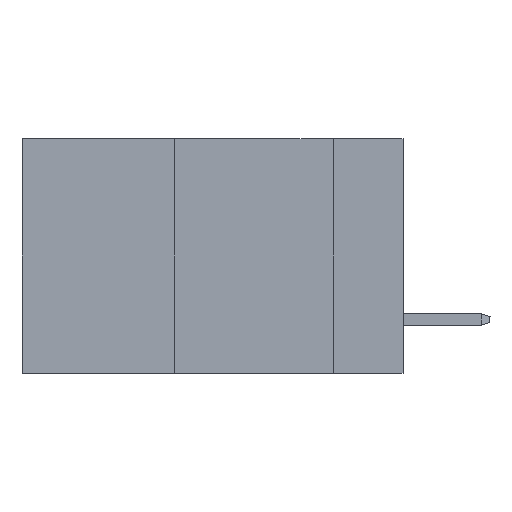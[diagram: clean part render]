
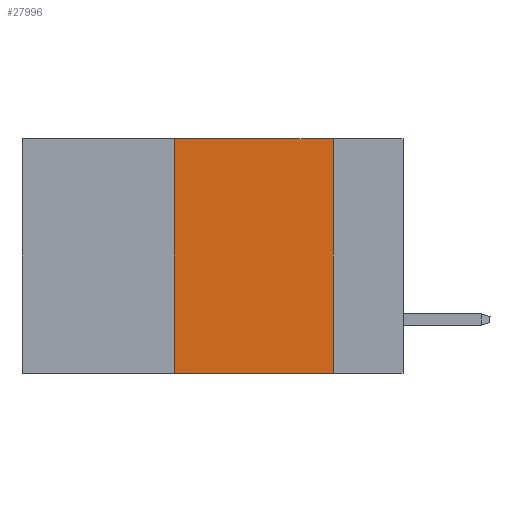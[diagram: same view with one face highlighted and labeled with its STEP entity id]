
A CAD part, left-side view. The second image highlights one B-rep face of the part: STEP entity #27996.
In plain terms, the highlighted planar face has unit normal (-1, 0, 0).
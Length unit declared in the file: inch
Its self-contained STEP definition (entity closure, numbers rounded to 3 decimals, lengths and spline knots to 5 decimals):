
#1361 = EDGE_CURVE ( 'NONE', #14462, #41740, #31360, .T. ) ;
#6105 = VECTOR ( 'NONE', #28665, 39.37008 ) ;
#7190 = LINE ( 'NONE', #13065, #34862 ) ;
#11686 = VECTOR ( 'NONE', #42303, 39.37008 ) ;
#12021 = EDGE_CURVE ( 'NONE', #26013, #41740, #7190, .T. ) ;
#13065 = CARTESIAN_POINT ( 'NONE',  ( 0., 0.6, -0.37 ) ) ;
#13126 = CARTESIAN_POINT ( 'NONE',  ( 0., 0.36, 0. ) ) ;
#14462 = VERTEX_POINT ( 'NONE', #42915 ) ;
#15807 = CARTESIAN_POINT ( 'NONE',  ( 0., 0.6, 0. ) ) ;
#17053 = CARTESIAN_POINT ( 'NONE',  ( 0., 0.36, 0. ) ) ;
#17493 = CARTESIAN_POINT ( 'NONE',  ( 0., 0.36, -0.37 ) ) ;
#18672 = CARTESIAN_POINT ( 'NONE',  ( 0., 0.11, -0.37 ) ) ;
#21296 = EDGE_CURVE ( 'NONE', #35274, #14462, #32718, .T. ) ;
#22016 = CARTESIAN_POINT ( 'NONE',  ( 0., 0.11, 0. ) ) ;
#22756 = PLANE ( 'NONE',  #42737 ) ;
#23080 = DIRECTION ( 'NONE',  ( 0., -1., 0. ) ) ;
#23664 = EDGE_LOOP ( 'NONE', ( #32026, #39330, #31536, #39510 ) ) ;
#25156 = DIRECTION ( 'NONE',  ( 1., 0., 0. ) ) ;
#26013 = VERTEX_POINT ( 'NONE', #17493 ) ;
#27851 = CARTESIAN_POINT ( 'NONE',  ( 0., 0.6, 0. ) ) ;
#27996 = ADVANCED_FACE ( 'NONE', ( #32481 ), #22756, .F. ) ;
#28665 = DIRECTION ( 'NONE',  ( 0., 0., 1. ) ) ;
#31360 = LINE ( 'NONE', #22016, #39396 ) ;
#31536 = ORIENTED_EDGE ( 'NONE', *, *, #38829, .F. ) ;
#32026 = ORIENTED_EDGE ( 'NONE', *, *, #1361, .F. ) ;
#32481 = FACE_OUTER_BOUND ( 'NONE', #23664, .T. ) ;
#32718 = LINE ( 'NONE', #15807, #11686 ) ;
#32879 = LINE ( 'NONE', #13126, #6105 ) ;
#34799 = DIRECTION ( 'NONE',  ( 0., 0., -1. ) ) ;
#34862 = VECTOR ( 'NONE', #23080, 39.37008 ) ;
#35274 = VERTEX_POINT ( 'NONE', #17053 ) ;
#38829 = EDGE_CURVE ( 'NONE', #26013, #35274, #32879, .T. ) ;
#39330 = ORIENTED_EDGE ( 'NONE', *, *, #21296, .F. ) ;
#39396 = VECTOR ( 'NONE', #34799, 39.37008 ) ;
#39510 = ORIENTED_EDGE ( 'NONE', *, *, #12021, .T. ) ;
#41740 = VERTEX_POINT ( 'NONE', #18672 ) ;
#41855 = DIRECTION ( 'NONE',  ( 0., 0., -1. ) ) ;
#42303 = DIRECTION ( 'NONE',  ( 0., -1., 0. ) ) ;
#42737 = AXIS2_PLACEMENT_3D ( 'NONE', #27851, #25156, #41855 ) ;
#42915 = CARTESIAN_POINT ( 'NONE',  ( 0., 0.11, 0. ) ) ;
